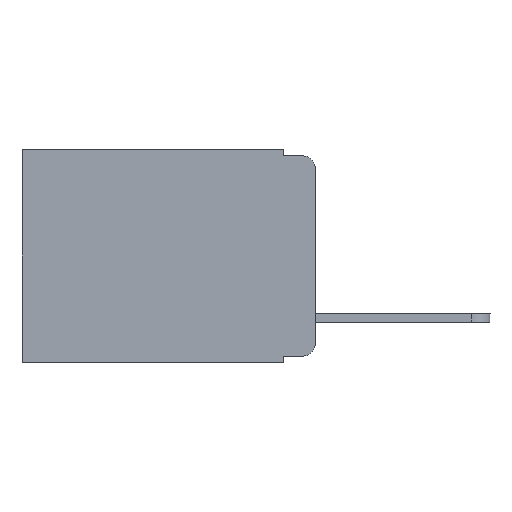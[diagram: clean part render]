
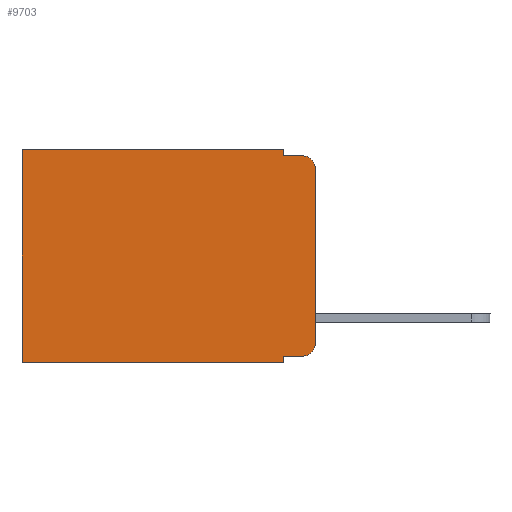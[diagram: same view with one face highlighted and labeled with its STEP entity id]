
A CAD part, left-side view. The second image highlights one B-rep face of the part: STEP entity #9703.
In plain terms, the highlighted planar face has unit normal (-1, 0, 0).
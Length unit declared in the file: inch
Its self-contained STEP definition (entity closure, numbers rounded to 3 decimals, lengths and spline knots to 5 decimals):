
#127 = CARTESIAN_POINT ( 'NONE',  ( 0.298, 0., 0. ) ) ;
#180 = VERTEX_POINT ( 'NONE', #4368 ) ;
#258 = CARTESIAN_POINT ( 'NONE',  ( 0.298, 0.051, -0.333 ) ) ;
#351 = LINE ( 'NONE', #127, #9799 ) ;
#369 = CIRCLE ( 'NONE', #7705, 0.02 ) ;
#454 = EDGE_CURVE ( 'NONE', #4975, #2359, #3870, .T. ) ;
#543 = DIRECTION ( 'NONE',  ( 0., -1., 0. ) ) ;
#799 = VERTEX_POINT ( 'NONE', #9687 ) ;
#959 = ORIENTED_EDGE ( 'NONE', *, *, #6560, .T. ) ;
#1052 = ORIENTED_EDGE ( 'NONE', *, *, #9930, .F. ) ;
#1146 = EDGE_CURVE ( 'NONE', #4975, #9211, #3740, .T. ) ;
#1549 = VECTOR ( 'NONE', #5343, 39.37008 ) ;
#1580 = VECTOR ( 'NONE', #6207, 39.37008 ) ;
#1705 = VECTOR ( 'NONE', #8348, 39.37008 ) ;
#1734 = CARTESIAN_POINT ( 'NONE',  ( 0.298, 0.051, -0.343 ) ) ;
#1899 = ORIENTED_EDGE ( 'NONE', *, *, #454, .F. ) ;
#2095 = CARTESIAN_POINT ( 'NONE',  ( 0.298, 0.051, -0.333 ) ) ;
#2103 = VERTEX_POINT ( 'NONE', #6256 ) ;
#2108 = DIRECTION ( 'NONE',  ( 0., 0., -1. ) ) ;
#2359 = VERTEX_POINT ( 'NONE', #1734 ) ;
#2514 = LINE ( 'NONE', #9567, #7331 ) ;
#2595 = EDGE_CURVE ( 'NONE', #3997, #9607, #5232, .T. ) ;
#2636 = VECTOR ( 'NONE', #5349, 39.37008 ) ;
#2684 = EDGE_CURVE ( 'NONE', #180, #4388, #369, .T. ) ;
#2762 = DIRECTION ( 'NONE',  ( 0., 0., -1. ) ) ;
#2863 = AXIS2_PLACEMENT_3D ( 'NONE', #9237, #6128, #6154 ) ;
#2869 = DIRECTION ( 'NONE',  ( -1., 0., 0. ) ) ;
#2877 = EDGE_CURVE ( 'NONE', #180, #2103, #351, .T. ) ;
#2904 = EDGE_LOOP ( 'NONE', ( #4500, #4374, #3556, #8449, #8361, #7843, #1052, #1899, #9866, #959 ) ) ;
#2976 = CARTESIAN_POINT ( 'NONE',  ( 0.298, 0.051, -0.01 ) ) ;
#3051 = VECTOR ( 'NONE', #2762, 39.37008 ) ;
#3556 = ORIENTED_EDGE ( 'NONE', *, *, #9292, .F. ) ;
#3740 = LINE ( 'NONE', #2095, #8902 ) ;
#3787 = DIRECTION ( 'NONE',  ( 0., 0., -1. ) ) ;
#3870 = LINE ( 'NONE', #9101, #1705 ) ;
#3997 = VERTEX_POINT ( 'NONE', #4138 ) ;
#4138 = CARTESIAN_POINT ( 'NONE',  ( 0.298, 0.051, 0. ) ) ;
#4368 = CARTESIAN_POINT ( 'NONE',  ( 0.298, 0., -0.03 ) ) ;
#4374 = ORIENTED_EDGE ( 'NONE', *, *, #2684, .T. ) ;
#4388 = VERTEX_POINT ( 'NONE', #8194 ) ;
#4420 = LINE ( 'NONE', #7552, #1549 ) ;
#4496 = CARTESIAN_POINT ( 'NONE',  ( 0.298, 0.473, -0.343 ) ) ;
#4500 = ORIENTED_EDGE ( 'NONE', *, *, #2877, .F. ) ;
#4593 = CARTESIAN_POINT ( 'NONE',  ( 0.298, 0., -0.343 ) ) ;
#4638 = CARTESIAN_POINT ( 'NONE',  ( 0.298, 0.051, -0.01 ) ) ;
#4975 = VERTEX_POINT ( 'NONE', #258 ) ;
#5232 = LINE ( 'NONE', #6662, #3051 ) ;
#5343 = DIRECTION ( 'NONE',  ( 0., 0., -1. ) ) ;
#5349 = DIRECTION ( 'NONE',  ( 0., 1., 0. ) ) ;
#5561 = DIRECTION ( 'NONE',  ( 0., 0., -1. ) ) ;
#5643 = EDGE_CURVE ( 'NONE', #3997, #799, #2514, .T. ) ;
#5673 = LINE ( 'NONE', #4638, #1580 ) ;
#5734 = DIRECTION ( 'NONE',  ( 0., 1., 0. ) ) ;
#6128 = DIRECTION ( 'NONE',  ( 1., 0., 0. ) ) ;
#6154 = DIRECTION ( 'NONE',  ( 0., 0., -1. ) ) ;
#6207 = DIRECTION ( 'NONE',  ( 0., -1., 0. ) ) ;
#6256 = CARTESIAN_POINT ( 'NONE',  ( 0.298, 0., -0.313 ) ) ;
#6470 = FACE_OUTER_BOUND ( 'NONE', #2904, .T. ) ;
#6473 = EDGE_CURVE ( 'NONE', #799, #9137, #4420, .T. ) ;
#6560 = EDGE_CURVE ( 'NONE', #9211, #2103, #6956, .T. ) ;
#6662 = CARTESIAN_POINT ( 'NONE',  ( 0.298, 0.051, 0. ) ) ;
#6687 = AXIS2_PLACEMENT_3D ( 'NONE', #9838, #2869, #2108 ) ;
#6800 = CARTESIAN_POINT ( 'NONE',  ( 0.298, 0.02, -0.03 ) ) ;
#6956 = CIRCLE ( 'NONE', #6687, 0.02 ) ;
#6985 = CARTESIAN_POINT ( 'NONE',  ( 0.298, 0.02, -0.333 ) ) ;
#7331 = VECTOR ( 'NONE', #5734, 39.37008 ) ;
#7552 = CARTESIAN_POINT ( 'NONE',  ( 0.298, 0.473, 0. ) ) ;
#7705 = AXIS2_PLACEMENT_3D ( 'NONE', #6800, #9918, #3787 ) ;
#7843 = ORIENTED_EDGE ( 'NONE', *, *, #6473, .T. ) ;
#8194 = CARTESIAN_POINT ( 'NONE',  ( 0.298, 0.02, -0.01 ) ) ;
#8348 = DIRECTION ( 'NONE',  ( 0., 0., -1. ) ) ;
#8361 = ORIENTED_EDGE ( 'NONE', *, *, #5643, .T. ) ;
#8449 = ORIENTED_EDGE ( 'NONE', *, *, #2595, .F. ) ;
#8902 = VECTOR ( 'NONE', #543, 39.37008 ) ;
#9101 = CARTESIAN_POINT ( 'NONE',  ( 0.298, 0.051, 0. ) ) ;
#9137 = VERTEX_POINT ( 'NONE', #4496 ) ;
#9211 = VERTEX_POINT ( 'NONE', #6985 ) ;
#9237 = CARTESIAN_POINT ( 'NONE',  ( 0.298, 0., 0. ) ) ;
#9292 = EDGE_CURVE ( 'NONE', #9607, #4388, #5673, .T. ) ;
#9567 = CARTESIAN_POINT ( 'NONE',  ( 0.298, 0., 0. ) ) ;
#9607 = VERTEX_POINT ( 'NONE', #2976 ) ;
#9687 = CARTESIAN_POINT ( 'NONE',  ( 0.298, 0.473, 0. ) ) ;
#9703 = ADVANCED_FACE ( 'NONE', ( #6470 ), #9944, .F. ) ;
#9752 = LINE ( 'NONE', #4593, #2636 ) ;
#9799 = VECTOR ( 'NONE', #5561, 39.37008 ) ;
#9838 = CARTESIAN_POINT ( 'NONE',  ( 0.298, 0.02, -0.313 ) ) ;
#9866 = ORIENTED_EDGE ( 'NONE', *, *, #1146, .T. ) ;
#9918 = DIRECTION ( 'NONE',  ( -1., 0., 0. ) ) ;
#9930 = EDGE_CURVE ( 'NONE', #2359, #9137, #9752, .T. ) ;
#9944 = PLANE ( 'NONE',  #2863 ) ;
